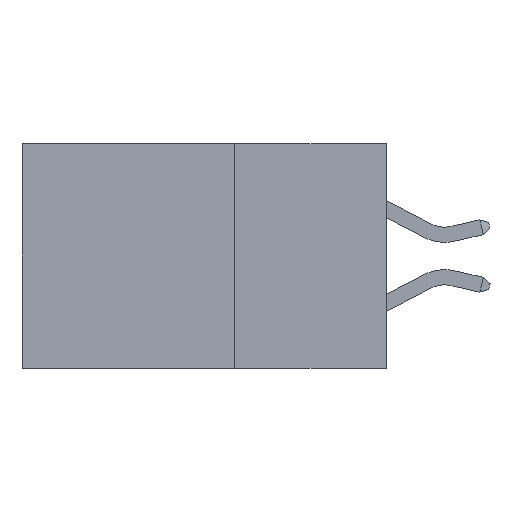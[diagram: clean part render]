
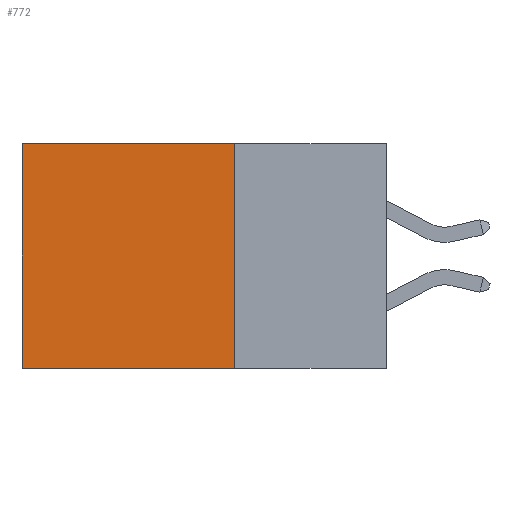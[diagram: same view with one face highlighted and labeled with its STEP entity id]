
A CAD part, left-side view. The second image highlights one B-rep face of the part: STEP entity #772.
In plain terms, the highlighted planar face has unit normal (-1, 0, 0).
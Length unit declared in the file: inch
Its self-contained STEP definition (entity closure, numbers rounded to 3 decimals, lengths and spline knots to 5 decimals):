
#107 = CARTESIAN_POINT ( 'NONE',  ( 0.298, 0.6, 0. ) ) ;
#772 = ADVANCED_FACE ( 'NONE', ( #4257 ), #13360, .F. ) ;
#1062 = LINE ( 'NONE', #10457, #16211 ) ;
#1256 = DIRECTION ( 'NONE',  ( 0., 0., -1. ) ) ;
#1309 = VECTOR ( 'NONE', #4684, 39.37008 ) ;
#1396 = DIRECTION ( 'NONE',  ( 1., 0., 0. ) ) ;
#2075 = EDGE_CURVE ( 'NONE', #3048, #14042, #9004, .T. ) ;
#2651 = AXIS2_PLACEMENT_3D ( 'NONE', #7222, #1396, #1256 ) ;
#3048 = VERTEX_POINT ( 'NONE', #4064 ) ;
#3075 = LINE ( 'NONE', #17918, #7102 ) ;
#4064 = CARTESIAN_POINT ( 'NONE',  ( 0.298, 0.25, 0. ) ) ;
#4257 = FACE_OUTER_BOUND ( 'NONE', #7159, .T. ) ;
#4684 = DIRECTION ( 'NONE',  ( 0., 1., 0. ) ) ;
#5898 = DIRECTION ( 'NONE',  ( 0., 0., -1. ) ) ;
#6495 = CARTESIAN_POINT ( 'NONE',  ( 0.298, 0.25, -0.37 ) ) ;
#7102 = VECTOR ( 'NONE', #13983, 39.37008 ) ;
#7159 = EDGE_LOOP ( 'NONE', ( #9340, #14618, #11246, #19566 ) ) ;
#7222 = CARTESIAN_POINT ( 'NONE',  ( 0.298, 0.25, 0. ) ) ;
#9004 = LINE ( 'NONE', #15500, #1309 ) ;
#9340 = ORIENTED_EDGE ( 'NONE', *, *, #13865, .T. ) ;
#9469 = EDGE_CURVE ( 'NONE', #10695, #10338, #17971, .T. ) ;
#9789 = CARTESIAN_POINT ( 'NONE',  ( 0.298, 0.25, -0.37 ) ) ;
#10338 = VERTEX_POINT ( 'NONE', #15276 ) ;
#10457 = CARTESIAN_POINT ( 'NONE',  ( 0.298, 0.25, 0. ) ) ;
#10695 = VERTEX_POINT ( 'NONE', #6495 ) ;
#11246 = ORIENTED_EDGE ( 'NONE', *, *, #18781, .F. ) ;
#13360 = PLANE ( 'NONE',  #2651 ) ;
#13663 = VECTOR ( 'NONE', #17688, 39.37008 ) ;
#13865 = EDGE_CURVE ( 'NONE', #14042, #10338, #3075, .T. ) ;
#13983 = DIRECTION ( 'NONE',  ( 0., 0., -1. ) ) ;
#14042 = VERTEX_POINT ( 'NONE', #107 ) ;
#14618 = ORIENTED_EDGE ( 'NONE', *, *, #9469, .F. ) ;
#15276 = CARTESIAN_POINT ( 'NONE',  ( 0.298, 0.6, -0.37 ) ) ;
#15500 = CARTESIAN_POINT ( 'NONE',  ( 0.298, 0.25, 0. ) ) ;
#16211 = VECTOR ( 'NONE', #5898, 39.37008 ) ;
#17688 = DIRECTION ( 'NONE',  ( 0., 1., 0. ) ) ;
#17918 = CARTESIAN_POINT ( 'NONE',  ( 0.298, 0.6, 0. ) ) ;
#17971 = LINE ( 'NONE', #9789, #13663 ) ;
#18781 = EDGE_CURVE ( 'NONE', #3048, #10695, #1062, .T. ) ;
#19566 = ORIENTED_EDGE ( 'NONE', *, *, #2075, .T. ) ;
